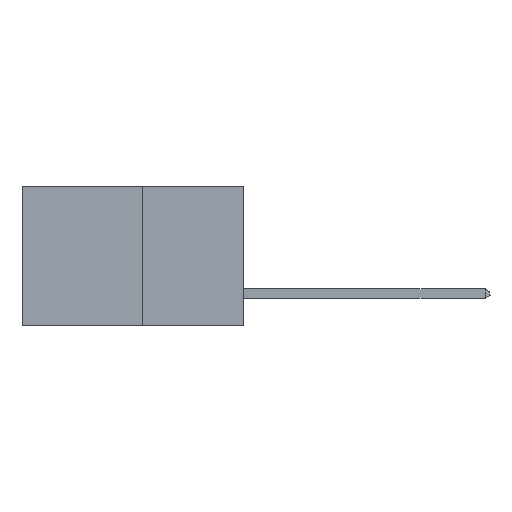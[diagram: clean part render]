
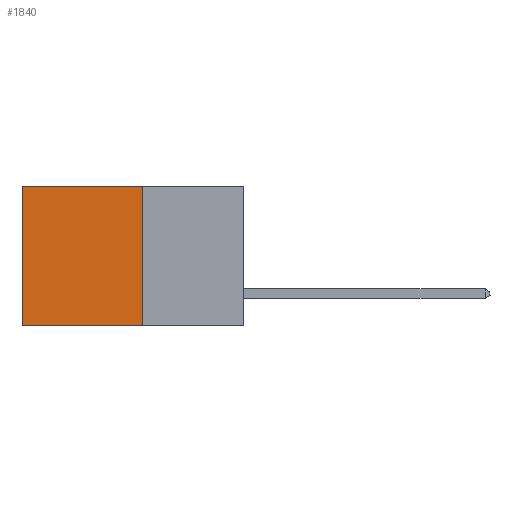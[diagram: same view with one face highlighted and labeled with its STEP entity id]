
A CAD part, left-side view. The second image highlights one B-rep face of the part: STEP entity #1840.
In plain terms, the highlighted planar face has unit normal (-1, 0, 0).
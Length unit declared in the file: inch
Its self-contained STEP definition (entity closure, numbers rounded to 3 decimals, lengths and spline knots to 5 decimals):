
#527 = VERTEX_POINT ( 'NONE', #1852 ) ;
#1143 = DIRECTION ( 'NONE',  ( 0., 1., 0. ) ) ;
#1163 = AXIS2_PLACEMENT_3D ( 'NONE', #14061, #14391, #2724 ) ;
#1590 = VECTOR ( 'NONE', #1143, 39.37008 ) ;
#1840 = ADVANCED_FACE ( 'NONE', ( #12298 ), #11139, .F. ) ;
#1852 = CARTESIAN_POINT ( 'NONE',  ( 0.277, 0.27, 0. ) ) ;
#2724 = DIRECTION ( 'NONE',  ( 0., 0., -1. ) ) ;
#2921 = ORIENTED_EDGE ( 'NONE', *, *, #11331, .T. ) ;
#3018 = LINE ( 'NONE', #10032, #11754 ) ;
#4097 = VERTEX_POINT ( 'NONE', #7579 ) ;
#4355 = EDGE_CURVE ( 'NONE', #527, #7893, #3018, .T. ) ;
#5355 = ORIENTED_EDGE ( 'NONE', *, *, #10425, .T. ) ;
#5457 = CARTESIAN_POINT ( 'NONE',  ( 0.277, 0.59, -0.37 ) ) ;
#5878 = ORIENTED_EDGE ( 'NONE', *, *, #10048, .F. ) ;
#6586 = ORIENTED_EDGE ( 'NONE', *, *, #4355, .F. ) ;
#7023 = CARTESIAN_POINT ( 'NONE',  ( 0.277, 0.27, 0. ) ) ;
#7579 = CARTESIAN_POINT ( 'NONE',  ( 0.277, 0.59, 0. ) ) ;
#7672 = DIRECTION ( 'NONE',  ( 0., 0., -1. ) ) ;
#7893 = VERTEX_POINT ( 'NONE', #13554 ) ;
#8076 = VECTOR ( 'NONE', #9102, 39.37008 ) ;
#8203 = EDGE_LOOP ( 'NONE', ( #5355, #5878, #6586, #2921 ) ) ;
#8410 = LINE ( 'NONE', #12036, #13974 ) ;
#8878 = VERTEX_POINT ( 'NONE', #5457 ) ;
#9102 = DIRECTION ( 'NONE',  ( 0., 1., 0. ) ) ;
#9798 = LINE ( 'NONE', #7023, #1590 ) ;
#10032 = CARTESIAN_POINT ( 'NONE',  ( 0.277, 0.27, -0.37 ) ) ;
#10048 = EDGE_CURVE ( 'NONE', #7893, #8878, #13384, .T. ) ;
#10129 = DIRECTION ( 'NONE',  ( 0., 0., -1. ) ) ;
#10425 = EDGE_CURVE ( 'NONE', #4097, #8878, #8410, .T. ) ;
#11139 = PLANE ( 'NONE',  #1163 ) ;
#11331 = EDGE_CURVE ( 'NONE', #527, #4097, #9798, .T. ) ;
#11754 = VECTOR ( 'NONE', #10129, 39.37008 ) ;
#12036 = CARTESIAN_POINT ( 'NONE',  ( 0.277, 0.59, -0.37 ) ) ;
#12298 = FACE_OUTER_BOUND ( 'NONE', #8203, .T. ) ;
#13384 = LINE ( 'NONE', #14266, #8076 ) ;
#13554 = CARTESIAN_POINT ( 'NONE',  ( 0.277, 0.27, -0.37 ) ) ;
#13974 = VECTOR ( 'NONE', #7672, 39.37008 ) ;
#14061 = CARTESIAN_POINT ( 'NONE',  ( 0.277, 0.27, -0.37 ) ) ;
#14266 = CARTESIAN_POINT ( 'NONE',  ( 0.277, 0.27, -0.37 ) ) ;
#14391 = DIRECTION ( 'NONE',  ( 1., 0., 0. ) ) ;
